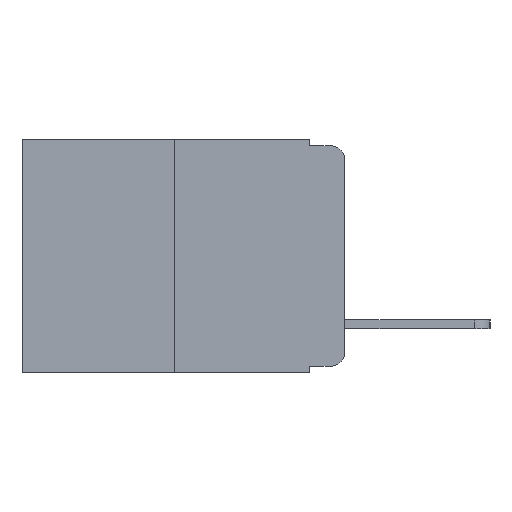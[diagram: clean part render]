
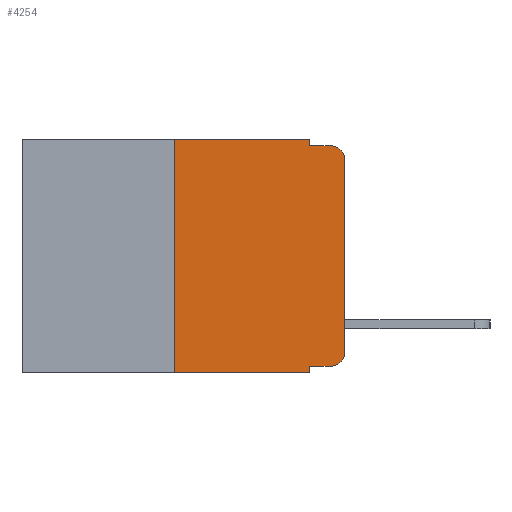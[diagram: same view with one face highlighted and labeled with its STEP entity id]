
A CAD part, left-side view. The second image highlights one B-rep face of the part: STEP entity #4254.
In plain terms, the highlighted planar face has unit normal (-1, 0, 0).
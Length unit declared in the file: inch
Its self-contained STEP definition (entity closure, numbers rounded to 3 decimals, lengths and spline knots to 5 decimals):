
#212 = AXIS2_PLACEMENT_3D ( 'NONE', #16890, #15480, #1660 ) ;
#253 = CARTESIAN_POINT ( 'NONE',  ( 0., 0.25, 0. ) ) ;
#257 = PLANE ( 'NONE',  #212 ) ;
#553 = VERTEX_POINT ( 'NONE', #12851 ) ;
#725 = ORIENTED_EDGE ( 'NONE', *, *, #8200, .F. ) ;
#1178 = ORIENTED_EDGE ( 'NONE', *, *, #4243, .T. ) ;
#1660 = DIRECTION ( 'NONE',  ( 0., 0., -1. ) ) ;
#1791 = CARTESIAN_POINT ( 'NONE',  ( 0., 0., -0.313 ) ) ;
#2103 = EDGE_LOOP ( 'NONE', ( #4976, #11779, #9871, #14274, #14910, #725, #14929, #3118, #1178, #17225 ) ) ;
#3108 = LINE ( 'NONE', #10362, #17407 ) ;
#3118 = ORIENTED_EDGE ( 'NONE', *, *, #6262, .F. ) ;
#3327 = DIRECTION ( 'NONE',  ( 0., -1., 0. ) ) ;
#3430 = CARTESIAN_POINT ( 'NONE',  ( 0., 0.02, -0.03 ) ) ;
#3517 = VECTOR ( 'NONE', #5556, 39.37008 ) ;
#3581 = CARTESIAN_POINT ( 'NONE',  ( 0., 0.02, -0.333 ) ) ;
#3849 = LINE ( 'NONE', #11545, #7368 ) ;
#4051 = CARTESIAN_POINT ( 'NONE',  ( 0., 0.051, -0.01 ) ) ;
#4057 = CARTESIAN_POINT ( 'NONE',  ( 0., 0.25, -0.343 ) ) ;
#4243 = EDGE_CURVE ( 'NONE', #15832, #14269, #3849, .T. ) ;
#4254 = ADVANCED_FACE ( 'NONE', ( #11058 ), #257, .F. ) ;
#4346 = DIRECTION ( 'NONE',  ( 0., -1., 0. ) ) ;
#4380 = VERTEX_POINT ( 'NONE', #4859 ) ;
#4817 = CARTESIAN_POINT ( 'NONE',  ( 0., 0.051, -0.343 ) ) ;
#4859 = CARTESIAN_POINT ( 'NONE',  ( 0., 0.02, -0.01 ) ) ;
#4895 = DIRECTION ( 'NONE',  ( 0., 0., -1. ) ) ;
#4930 = VECTOR ( 'NONE', #8658, 39.37008 ) ;
#4976 = ORIENTED_EDGE ( 'NONE', *, *, #7167, .T. ) ;
#4977 = VERTEX_POINT ( 'NONE', #4057 ) ;
#5295 = AXIS2_PLACEMENT_3D ( 'NONE', #3430, #13328, #4895 ) ;
#5556 = DIRECTION ( 'NONE',  ( 0., -1., 0. ) ) ;
#5559 = CARTESIAN_POINT ( 'NONE',  ( 0., 0.25, 0. ) ) ;
#6262 = EDGE_CURVE ( 'NONE', #15832, #13406, #13744, .T. ) ;
#6831 = VECTOR ( 'NONE', #8501, 39.37008 ) ;
#7033 = VECTOR ( 'NONE', #3327, 39.37008 ) ;
#7167 = EDGE_CURVE ( 'NONE', #13303, #14240, #9681, .T. ) ;
#7256 = VERTEX_POINT ( 'NONE', #253 ) ;
#7368 = VECTOR ( 'NONE', #4346, 39.37008 ) ;
#7406 = CARTESIAN_POINT ( 'NONE',  ( 0., 0.051, 0. ) ) ;
#8200 = EDGE_CURVE ( 'NONE', #4977, #7256, #17613, .T. ) ;
#8215 = DIRECTION ( 'NONE',  ( -1., 0., 0. ) ) ;
#8501 = DIRECTION ( 'NONE',  ( 0., 0., 1. ) ) ;
#8658 = DIRECTION ( 'NONE',  ( 0., 0., 1. ) ) ;
#8799 = EDGE_CURVE ( 'NONE', #4977, #13406, #11578, .T. ) ;
#9681 = LINE ( 'NONE', #16715, #4930 ) ;
#9762 = CIRCLE ( 'NONE', #10868, 0.02 ) ;
#9871 = ORIENTED_EDGE ( 'NONE', *, *, #15126, .F. ) ;
#10362 = CARTESIAN_POINT ( 'NONE',  ( 0., 0.473, 0. ) ) ;
#10736 = EDGE_CURVE ( 'NONE', #14269, #13303, #9762, .T. ) ;
#10868 = AXIS2_PLACEMENT_3D ( 'NONE', #16287, #8215, #17631 ) ;
#11058 = FACE_OUTER_BOUND ( 'NONE', #2103, .T. ) ;
#11080 = CARTESIAN_POINT ( 'NONE',  ( 0., 0.051, 0. ) ) ;
#11165 = LINE ( 'NONE', #4051, #3517 ) ;
#11545 = CARTESIAN_POINT ( 'NONE',  ( 0., 0.051, -0.333 ) ) ;
#11578 = LINE ( 'NONE', #17153, #7033 ) ;
#11779 = ORIENTED_EDGE ( 'NONE', *, *, #16912, .T. ) ;
#12259 = VECTOR ( 'NONE', #12436, 39.37008 ) ;
#12436 = DIRECTION ( 'NONE',  ( 0., 0., -1. ) ) ;
#12851 = CARTESIAN_POINT ( 'NONE',  ( 0., 0.051, -0.01 ) ) ;
#13303 = VERTEX_POINT ( 'NONE', #1791 ) ;
#13328 = DIRECTION ( 'NONE',  ( -1., 0., 0. ) ) ;
#13406 = VERTEX_POINT ( 'NONE', #4817 ) ;
#13686 = EDGE_CURVE ( 'NONE', #17217, #553, #15770, .T. ) ;
#13744 = LINE ( 'NONE', #7406, #15992 ) ;
#13766 = CARTESIAN_POINT ( 'NONE',  ( 0., 0.051, -0.333 ) ) ;
#14240 = VERTEX_POINT ( 'NONE', #14723 ) ;
#14269 = VERTEX_POINT ( 'NONE', #3581 ) ;
#14274 = ORIENTED_EDGE ( 'NONE', *, *, #13686, .F. ) ;
#14413 = DIRECTION ( 'NONE',  ( 0., -1., 0. ) ) ;
#14599 = EDGE_CURVE ( 'NONE', #7256, #17217, #3108, .T. ) ;
#14723 = CARTESIAN_POINT ( 'NONE',  ( 0., 0., -0.03 ) ) ;
#14910 = ORIENTED_EDGE ( 'NONE', *, *, #14599, .F. ) ;
#14929 = ORIENTED_EDGE ( 'NONE', *, *, #8799, .T. ) ;
#15126 = EDGE_CURVE ( 'NONE', #553, #4380, #11165, .T. ) ;
#15222 = CARTESIAN_POINT ( 'NONE',  ( 0., 0.051, 0. ) ) ;
#15480 = DIRECTION ( 'NONE',  ( 1., 0., 0. ) ) ;
#15526 = DIRECTION ( 'NONE',  ( 0., 0., -1. ) ) ;
#15770 = LINE ( 'NONE', #11080, #12259 ) ;
#15832 = VERTEX_POINT ( 'NONE', #13766 ) ;
#15992 = VECTOR ( 'NONE', #15526, 39.37008 ) ;
#16164 = CIRCLE ( 'NONE', #5295, 0.02 ) ;
#16287 = CARTESIAN_POINT ( 'NONE',  ( 0., 0.02, -0.313 ) ) ;
#16715 = CARTESIAN_POINT ( 'NONE',  ( 0., 0., 0. ) ) ;
#16890 = CARTESIAN_POINT ( 'NONE',  ( 0., 0.473, 0. ) ) ;
#16912 = EDGE_CURVE ( 'NONE', #14240, #4380, #16164, .T. ) ;
#17153 = CARTESIAN_POINT ( 'NONE',  ( 0., 0.473, -0.343 ) ) ;
#17217 = VERTEX_POINT ( 'NONE', #15222 ) ;
#17225 = ORIENTED_EDGE ( 'NONE', *, *, #10736, .T. ) ;
#17407 = VECTOR ( 'NONE', #14413, 39.37008 ) ;
#17613 = LINE ( 'NONE', #5559, #6831 ) ;
#17631 = DIRECTION ( 'NONE',  ( 0., 0., -1. ) ) ;
